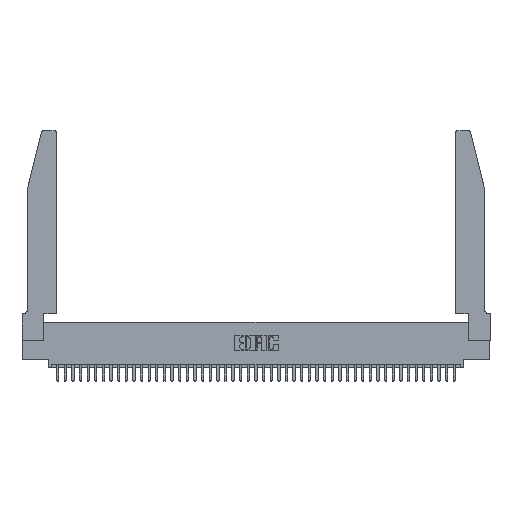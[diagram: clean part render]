
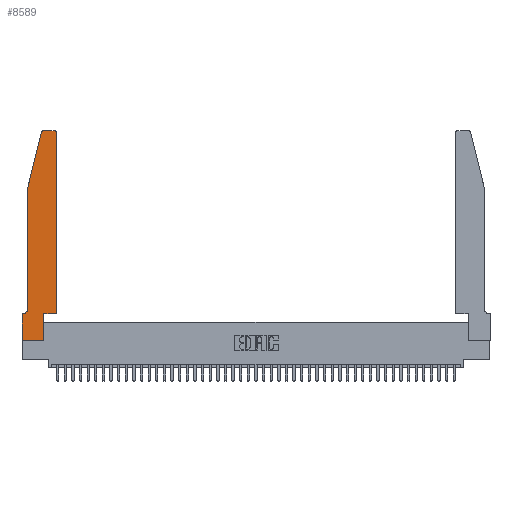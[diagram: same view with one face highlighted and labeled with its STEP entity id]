
A CAD part, top view. The second image highlights one B-rep face of the part: STEP entity #8589.
In plain terms, the highlighted planar face has unit normal (0, 0, 1).
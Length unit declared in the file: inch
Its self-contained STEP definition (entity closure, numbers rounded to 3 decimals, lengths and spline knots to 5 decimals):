
#749 = FACE_OUTER_BOUND ( 'NONE', #22443, .T. ) ;
#851 = ORIENTED_EDGE ( 'NONE', *, *, #32539, .T. ) ;
#1203 = DIRECTION ( 'NONE',  ( -0.239, -0.971, 0. ) ) ;
#2207 = CARTESIAN_POINT ( 'NONE',  ( 0.284, 2.75, 0.37 ) ) ;
#3036 = VERTEX_POINT ( 'NONE', #9545 ) ;
#3195 = DIRECTION ( 'NONE',  ( 1., 0., 0. ) ) ;
#4336 = ORIENTED_EDGE ( 'NONE', *, *, #44168, .T. ) ;
#4366 = CARTESIAN_POINT ( 'NONE',  ( 0.2865, 0.35, 0.37 ) ) ;
#4444 = VERTEX_POINT ( 'NONE', #18664 ) ;
#4786 = EDGE_CURVE ( 'NONE', #21933, #34284, #23720, .T. ) ;
#4892 = DIRECTION ( 'NONE',  ( 0., -1., 0. ) ) ;
#5269 = LINE ( 'NONE', #30943, #32123 ) ;
#5615 = VERTEX_POINT ( 'NONE', #31163 ) ;
#5862 = EDGE_CURVE ( 'NONE', #5615, #11201, #38175, .T. ) ;
#7064 = ORIENTED_EDGE ( 'NONE', *, *, #9316, .T. ) ;
#7578 = CARTESIAN_POINT ( 'NONE',  ( 0.4505, 0.35, 0.37 ) ) ;
#7628 = ORIENTED_EDGE ( 'NONE', *, *, #5862, .T. ) ;
#8194 = ORIENTED_EDGE ( 'NONE', *, *, #38554, .T. ) ;
#8589 = ADVANCED_FACE ( 'NONE', ( #749 ), #12624, .T. ) ;
#9108 = DIRECTION ( 'NONE',  ( 0., 0., 1. ) ) ;
#9316 = EDGE_CURVE ( 'NONE', #11856, #27525, #10487, .T. ) ;
#9329 = VECTOR ( 'NONE', #11080, 39.37008 ) ;
#9368 = VECTOR ( 'NONE', #40511, 39.37008 ) ;
#9545 = CARTESIAN_POINT ( 'NONE',  ( 0.4505, 0.35, 0.37 ) ) ;
#10108 = DIRECTION ( 'NONE',  ( 0., 0., 1. ) ) ;
#10487 = LINE ( 'NONE', #26686, #9368 ) ;
#10631 = CIRCLE ( 'NONE', #29792, 0.03 ) ;
#11080 = DIRECTION ( 'NONE',  ( 0., 1., 0. ) ) ;
#11201 = VERTEX_POINT ( 'NONE', #37947 ) ;
#11856 = VERTEX_POINT ( 'NONE', #31550 ) ;
#12624 = PLANE ( 'NONE',  #26066 ) ;
#13536 = DIRECTION ( 'NONE',  ( 0., -1., 0. ) ) ;
#13787 = CIRCLE ( 'NONE', #30556, 0.03 ) ;
#13916 = CARTESIAN_POINT ( 'NONE',  ( 0.25487, 2.72718, 0.37 ) ) ;
#14565 = VECTOR ( 'NONE', #22073, 39.37008 ) ;
#14664 = EDGE_CURVE ( 'NONE', #40496, #5615, #41289, .T. ) ;
#14936 = DIRECTION ( 'NONE',  ( 0., 1., 0. ) ) ;
#15447 = EDGE_CURVE ( 'NONE', #34284, #39738, #10631, .T. ) ;
#16034 = LINE ( 'NONE', #22155, #33544 ) ;
#16153 = DIRECTION ( 'NONE',  ( 0., 0., 1. ) ) ;
#16421 = LINE ( 'NONE', #25883, #33924 ) ;
#16616 = LINE ( 'NONE', #44958, #34116 ) ;
#16755 = ORIENTED_EDGE ( 'NONE', *, *, #22872, .T. ) ;
#18664 = CARTESIAN_POINT ( 'NONE',  ( 0.0755, 2., 0.37 ) ) ;
#19162 = ORIENTED_EDGE ( 'NONE', *, *, #30296, .T. ) ;
#20196 = DIRECTION ( 'NONE',  ( 0., 0., -1. ) ) ;
#20770 = ORIENTED_EDGE ( 'NONE', *, *, #15447, .T. ) ;
#21129 = VERTEX_POINT ( 'NONE', #42226 ) ;
#21933 = VERTEX_POINT ( 'NONE', #33371 ) ;
#22073 = DIRECTION ( 'NONE',  ( 1., 0., 0. ) ) ;
#22155 = CARTESIAN_POINT ( 'NONE',  ( 0.0755, 2., 0.37 ) ) ;
#22443 = EDGE_LOOP ( 'NONE', ( #38097, #20770, #30311, #43657, #4336, #7064, #19162, #35359, #7628, #16755, #8194, #851 ) ) ;
#22872 = EDGE_CURVE ( 'NONE', #11201, #3036, #16616, .T. ) ;
#23125 = EDGE_CURVE ( 'NONE', #39738, #4444, #16034, .T. ) ;
#23720 = LINE ( 'NONE', #24155, #36017 ) ;
#24155 = CARTESIAN_POINT ( 'NONE',  ( 0.2605, 2.75, 0.37 ) ) ;
#25883 = CARTESIAN_POINT ( 'NONE',  ( 0., 0., 0.37 ) ) ;
#26066 = AXIS2_PLACEMENT_3D ( 'NONE', #37110, #16153, #40563 ) ;
#26686 = CARTESIAN_POINT ( 'NONE',  ( 0.0755, 0.35, 0.37 ) ) ;
#27380 = CARTESIAN_POINT ( 'NONE',  ( 0., 0.35, 0.37 ) ) ;
#27525 = VERTEX_POINT ( 'NONE', #27380 ) ;
#28223 = CARTESIAN_POINT ( 'NONE',  ( 0., 0., 0.37 ) ) ;
#29792 = AXIS2_PLACEMENT_3D ( 'NONE', #30105, #9108, #33602 ) ;
#30105 = CARTESIAN_POINT ( 'NONE',  ( 0.284, 2.72, 0.37 ) ) ;
#30296 = EDGE_CURVE ( 'NONE', #27525, #40496, #16421, .T. ) ;
#30311 = ORIENTED_EDGE ( 'NONE', *, *, #23125, .T. ) ;
#30556 = AXIS2_PLACEMENT_3D ( 'NONE', #31072, #10108, #34597 ) ;
#30943 = CARTESIAN_POINT ( 'NONE',  ( 0.0755, 2., 0.37 ) ) ;
#31072 = CARTESIAN_POINT ( 'NONE',  ( 0.4205, 2.72, 0.37 ) ) ;
#31163 = CARTESIAN_POINT ( 'NONE',  ( 0.2865, 0., 0.37 ) ) ;
#31550 = CARTESIAN_POINT ( 'NONE',  ( 0.0055, 0.35, 0.37 ) ) ;
#32123 = VECTOR ( 'NONE', #13536, 39.37008 ) ;
#32539 = EDGE_CURVE ( 'NONE', #21129, #21933, #13787, .T. ) ;
#33371 = CARTESIAN_POINT ( 'NONE',  ( 0.4205, 2.75, 0.37 ) ) ;
#33544 = VECTOR ( 'NONE', #1203, 39.37008 ) ;
#33602 = DIRECTION ( 'NONE',  ( 1., 0., 0. ) ) ;
#33924 = VECTOR ( 'NONE', #4892, 39.37008 ) ;
#34042 = CARTESIAN_POINT ( 'NONE',  ( 0.0755, 0.42, 0.37 ) ) ;
#34116 = VECTOR ( 'NONE', #3195, 39.37008 ) ;
#34284 = VERTEX_POINT ( 'NONE', #2207 ) ;
#34597 = DIRECTION ( 'NONE',  ( 1., 0., 0. ) ) ;
#35359 = ORIENTED_EDGE ( 'NONE', *, *, #14664, .T. ) ;
#35521 = AXIS2_PLACEMENT_3D ( 'NONE', #41023, #20196, #44512 ) ;
#36017 = VECTOR ( 'NONE', #38005, 39.37008 ) ;
#37085 = VECTOR ( 'NONE', #14936, 39.37008 ) ;
#37110 = CARTESIAN_POINT ( 'NONE',  ( 0., 0.35, 0.37 ) ) ;
#37272 = LINE ( 'NONE', #7578, #9329 ) ;
#37947 = CARTESIAN_POINT ( 'NONE',  ( 0.2865, 0.35, 0.37 ) ) ;
#38005 = DIRECTION ( 'NONE',  ( -1., 0., 0. ) ) ;
#38097 = ORIENTED_EDGE ( 'NONE', *, *, #4786, .T. ) ;
#38175 = LINE ( 'NONE', #4366, #37085 ) ;
#38554 = EDGE_CURVE ( 'NONE', #3036, #21129, #37272, .T. ) ;
#39738 = VERTEX_POINT ( 'NONE', #13916 ) ;
#40258 = VERTEX_POINT ( 'NONE', #34042 ) ;
#40496 = VERTEX_POINT ( 'NONE', #28223 ) ;
#40511 = DIRECTION ( 'NONE',  ( -1., 0., 0. ) ) ;
#40563 = DIRECTION ( 'NONE',  ( 1., 0., 0. ) ) ;
#40835 = EDGE_CURVE ( 'NONE', #4444, #40258, #5269, .T. ) ;
#41023 = CARTESIAN_POINT ( 'NONE',  ( 0.0055, 0.42, 0.37 ) ) ;
#41289 = LINE ( 'NONE', #42892, #14565 ) ;
#42226 = CARTESIAN_POINT ( 'NONE',  ( 0.4505, 2.72, 0.37 ) ) ;
#42892 = CARTESIAN_POINT ( 'NONE',  ( 0., 0., 0.37 ) ) ;
#43657 = ORIENTED_EDGE ( 'NONE', *, *, #40835, .T. ) ;
#44168 = EDGE_CURVE ( 'NONE', #40258, #11856, #44285, .T. ) ;
#44285 = CIRCLE ( 'NONE', #35521, 0.07 ) ;
#44512 = DIRECTION ( 'NONE',  ( -1., 0., 0. ) ) ;
#44958 = CARTESIAN_POINT ( 'NONE',  ( 0.4505, 0.35, 0.37 ) ) ;
